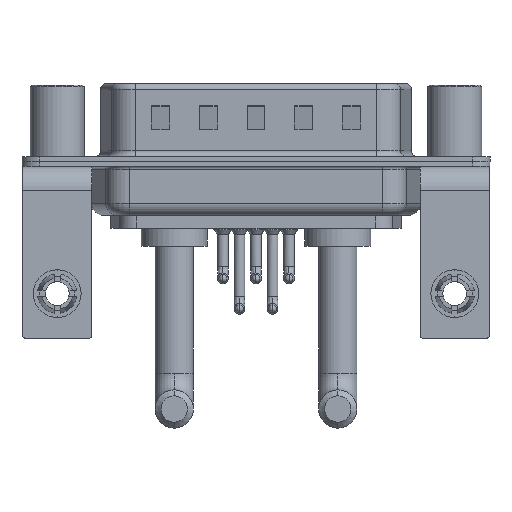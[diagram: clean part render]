
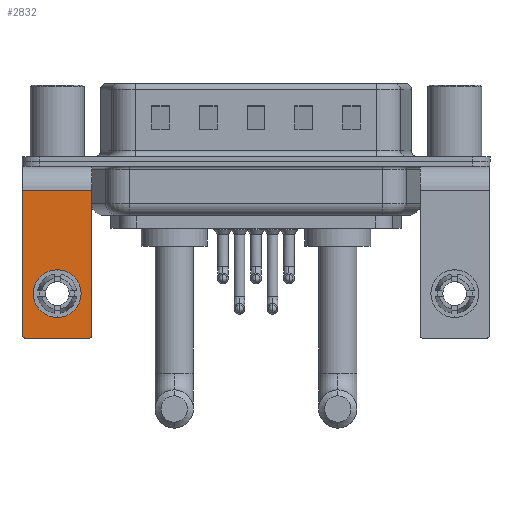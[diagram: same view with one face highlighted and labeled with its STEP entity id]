
A CAD part, front view. The second image highlights one B-rep face of the part: STEP entity #2832.
In plain terms, the highlighted planar face has unit normal (0, -1, 0).
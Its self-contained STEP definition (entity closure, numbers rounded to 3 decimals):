
#478 = CARTESIAN_POINT ( 'NONE',  ( -2.9, -6.25, -14.55 ) ) ;
#514 = DIRECTION ( 'NONE',  ( 0., 0., 1. ) ) ;
#600 = CARTESIAN_POINT ( 'NONE',  ( 0., -6.25, -11.07 ) ) ;
#851 = DIRECTION ( 'NONE',  ( 0., -1., 0. ) ) ;
#1395 = ORIENTED_EDGE ( 'NONE', *, *, #8468, .F. ) ;
#1824 = CIRCLE ( 'NONE', #2625, 0.25 ) ;
#2001 = CARTESIAN_POINT ( 'NONE',  ( 2.9, -6.25, -2.4 ) ) ;
#2131 = EDGE_CURVE ( 'NONE', #5889, #19667, #13200, .T. ) ;
#2379 = DIRECTION ( 'NONE',  ( 0., -1., 0. ) ) ;
#2591 = CARTESIAN_POINT ( 'NONE',  ( 2.65, -6.25, -14.8 ) ) ;
#2619 = DIRECTION ( 'NONE',  ( 0., 0., 1. ) ) ;
#2625 = AXIS2_PLACEMENT_3D ( 'NONE', #22156, #851, #19755 ) ;
#2832 = ADVANCED_FACE ( 'NONE', ( #12489, #8929 ), #20211, .F. ) ;
#3814 = CARTESIAN_POINT ( 'NONE',  ( 2.9, -6.25, -14.55 ) ) ;
#3825 = EDGE_LOOP ( 'NONE', ( #14706, #12501 ) ) ;
#4042 = VERTEX_POINT ( 'NONE', #2591 ) ;
#4166 = CARTESIAN_POINT ( 'NONE',  ( -2.65, -6.25, -14.55 ) ) ;
#4167 = DIRECTION ( 'NONE',  ( 0., 1., 0. ) ) ;
#4663 = VECTOR ( 'NONE', #9745, 1000. ) ;
#4732 = EDGE_LOOP ( 'NONE', ( #12476, #11890, #1395, #22889, #17168, #17787 ) ) ;
#4807 = AXIS2_PLACEMENT_3D ( 'NONE', #600, #4167, #8347 ) ;
#4883 = CARTESIAN_POINT ( 'NONE',  ( -2.9, -6.25, -2.4 ) ) ;
#5428 = CARTESIAN_POINT ( 'NONE',  ( 0., -6.25, -9.07 ) ) ;
#5541 = EDGE_CURVE ( 'NONE', #13371, #5889, #22052, .T. ) ;
#5884 = EDGE_CURVE ( 'NONE', #22415, #19115, #6026, .T. ) ;
#5889 = VERTEX_POINT ( 'NONE', #478 ) ;
#6026 = CIRCLE ( 'NONE', #4807, 2. ) ;
#6150 = CARTESIAN_POINT ( 'NONE',  ( -2.65, -6.25, -14.8 ) ) ;
#6729 = CARTESIAN_POINT ( 'NONE',  ( -2.9, -6.25, -2.4 ) ) ;
#6780 = VERTEX_POINT ( 'NONE', #3814 ) ;
#7216 = EDGE_CURVE ( 'NONE', #22404, #6780, #13412, .T. ) ;
#7289 = EDGE_CURVE ( 'NONE', #4042, #6780, #1824, .T. ) ;
#8062 = LINE ( 'NONE', #16041, #18866 ) ;
#8084 = EDGE_CURVE ( 'NONE', #19115, #22415, #15635, .T. ) ;
#8347 = DIRECTION ( 'NONE',  ( 0., 0., 1. ) ) ;
#8468 = EDGE_CURVE ( 'NONE', #4042, #19667, #8062, .T. ) ;
#8929 = FACE_OUTER_BOUND ( 'NONE', #4732, .T. ) ;
#9745 = DIRECTION ( 'NONE',  ( 0., 0., -1. ) ) ;
#9898 = CARTESIAN_POINT ( 'NONE',  ( 2.9, -6.25, -2.4 ) ) ;
#10156 = CARTESIAN_POINT ( 'NONE',  ( 0., -6.25, -11.07 ) ) ;
#10585 = CARTESIAN_POINT ( 'NONE',  ( 2.9, -6.25, -2.4 ) ) ;
#10778 = AXIS2_PLACEMENT_3D ( 'NONE', #10156, #23840, #514 ) ;
#11890 = ORIENTED_EDGE ( 'NONE', *, *, #2131, .T. ) ;
#12429 = CARTESIAN_POINT ( 'NONE',  ( 2.9, -6.25, -2.4 ) ) ;
#12476 = ORIENTED_EDGE ( 'NONE', *, *, #5541, .T. ) ;
#12489 = FACE_BOUND ( 'NONE', #3825, .T. ) ;
#12501 = ORIENTED_EDGE ( 'NONE', *, *, #5884, .T. ) ;
#13200 = CIRCLE ( 'NONE', #19252, 0.25 ) ;
#13371 = VERTEX_POINT ( 'NONE', #4883 ) ;
#13412 = LINE ( 'NONE', #2001, #4663 ) ;
#14706 = ORIENTED_EDGE ( 'NONE', *, *, #8084, .T. ) ;
#15635 = CIRCLE ( 'NONE', #10778, 2. ) ;
#15728 = VECTOR ( 'NONE', #23958, 1000. ) ;
#15916 = DIRECTION ( 'NONE',  ( -1., 0., 0. ) ) ;
#16041 = CARTESIAN_POINT ( 'NONE',  ( 2.9, -6.25, -14.8 ) ) ;
#16185 = AXIS2_PLACEMENT_3D ( 'NONE', #10585, #24155, #22487 ) ;
#17168 = ORIENTED_EDGE ( 'NONE', *, *, #7216, .F. ) ;
#17371 = LINE ( 'NONE', #9898, #20422 ) ;
#17787 = ORIENTED_EDGE ( 'NONE', *, *, #20473, .T. ) ;
#18866 = VECTOR ( 'NONE', #15916, 1000. ) ;
#19115 = VERTEX_POINT ( 'NONE', #21166 ) ;
#19128 = DIRECTION ( 'NONE',  ( -1., 0., 0. ) ) ;
#19252 = AXIS2_PLACEMENT_3D ( 'NONE', #4166, #2379, #2619 ) ;
#19667 = VERTEX_POINT ( 'NONE', #6150 ) ;
#19755 = DIRECTION ( 'NONE',  ( 0., 0., 1. ) ) ;
#20211 = PLANE ( 'NONE',  #16185 ) ;
#20422 = VECTOR ( 'NONE', #19128, 1000. ) ;
#20473 = EDGE_CURVE ( 'NONE', #22404, #13371, #17371, .T. ) ;
#21166 = CARTESIAN_POINT ( 'NONE',  ( 0., -6.25, -13.07 ) ) ;
#22052 = LINE ( 'NONE', #6729, #15728 ) ;
#22156 = CARTESIAN_POINT ( 'NONE',  ( 2.65, -6.25, -14.55 ) ) ;
#22404 = VERTEX_POINT ( 'NONE', #12429 ) ;
#22415 = VERTEX_POINT ( 'NONE', #5428 ) ;
#22487 = DIRECTION ( 'NONE',  ( 0., 0., 1. ) ) ;
#22889 = ORIENTED_EDGE ( 'NONE', *, *, #7289, .T. ) ;
#23840 = DIRECTION ( 'NONE',  ( 0., 1., 0. ) ) ;
#23958 = DIRECTION ( 'NONE',  ( 0., 0., -1. ) ) ;
#24155 = DIRECTION ( 'NONE',  ( 0., 1., 0. ) ) ;
